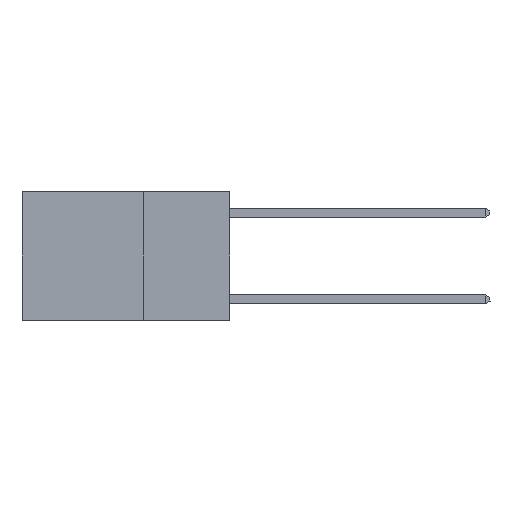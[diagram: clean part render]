
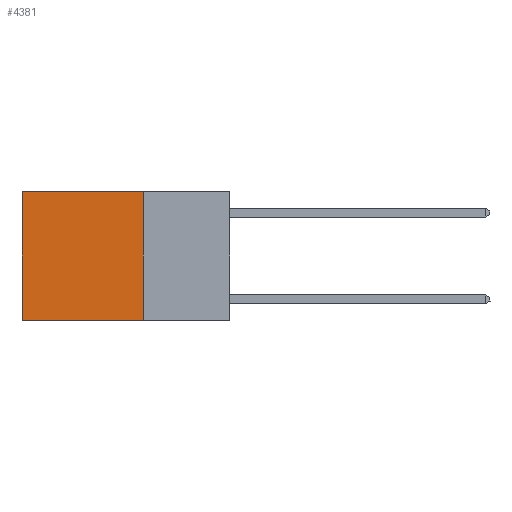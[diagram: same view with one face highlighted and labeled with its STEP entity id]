
A CAD part, left-side view. The second image highlights one B-rep face of the part: STEP entity #4381.
In plain terms, the highlighted planar face has unit normal (-1, 0, 0).
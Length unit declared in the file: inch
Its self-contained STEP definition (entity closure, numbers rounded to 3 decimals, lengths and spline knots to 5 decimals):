
#1529 = LINE ( 'NONE', #4087, #15041 ) ;
#1538 = VERTEX_POINT ( 'NONE', #12390 ) ;
#1832 = EDGE_CURVE ( 'NONE', #18325, #11572, #9475, .T. ) ;
#1994 = DIRECTION ( 'NONE',  ( 0., 0., -1. ) ) ;
#3915 = EDGE_LOOP ( 'NONE', ( #21281, #9006, #17291, #7920 ) ) ;
#4087 = CARTESIAN_POINT ( 'NONE',  ( 0.2625, 0.25, 0. ) ) ;
#4342 = CARTESIAN_POINT ( 'NONE',  ( 0.2625, 0.25, -0.37 ) ) ;
#4381 = ADVANCED_FACE ( 'NONE', ( #10712 ), #11889, .F. ) ;
#5297 = EDGE_CURVE ( 'NONE', #1538, #17849, #1529, .T. ) ;
#5968 = DIRECTION ( 'NONE',  ( 1., 0., 0. ) ) ;
#6280 = CARTESIAN_POINT ( 'NONE',  ( 0.2625, 0.25, -0.37 ) ) ;
#6551 = AXIS2_PLACEMENT_3D ( 'NONE', #14494, #5968, #1994 ) ;
#7920 = ORIENTED_EDGE ( 'NONE', *, *, #5297, .T. ) ;
#8120 = VECTOR ( 'NONE', #9567, 39.37008 ) ;
#9006 = ORIENTED_EDGE ( 'NONE', *, *, #1832, .F. ) ;
#9340 = LINE ( 'NONE', #21390, #16063 ) ;
#9475 = LINE ( 'NONE', #4342, #8120 ) ;
#9567 = DIRECTION ( 'NONE',  ( 0., 1., 0. ) ) ;
#10415 = CARTESIAN_POINT ( 'NONE',  ( 0.2625, 0.6, 0. ) ) ;
#10712 = FACE_OUTER_BOUND ( 'NONE', #3915, .T. ) ;
#10870 = VECTOR ( 'NONE', #11507, 39.37008 ) ;
#11131 = CARTESIAN_POINT ( 'NONE',  ( 0.2625, 0.6, -0.37 ) ) ;
#11487 = DIRECTION ( 'NONE',  ( 0., 0., -1. ) ) ;
#11507 = DIRECTION ( 'NONE',  ( 0., 0., -1. ) ) ;
#11572 = VERTEX_POINT ( 'NONE', #11131 ) ;
#11889 = PLANE ( 'NONE',  #6551 ) ;
#12390 = CARTESIAN_POINT ( 'NONE',  ( 0.2625, 0.25, 0. ) ) ;
#14466 = DIRECTION ( 'NONE',  ( 0., 1., 0. ) ) ;
#14494 = CARTESIAN_POINT ( 'NONE',  ( 0.2625, 0.25, 0. ) ) ;
#14552 = EDGE_CURVE ( 'NONE', #17849, #11572, #9340, .T. ) ;
#15041 = VECTOR ( 'NONE', #14466, 39.37008 ) ;
#16063 = VECTOR ( 'NONE', #11487, 39.37008 ) ;
#16964 = EDGE_CURVE ( 'NONE', #1538, #18325, #21074, .T. ) ;
#17291 = ORIENTED_EDGE ( 'NONE', *, *, #16964, .F. ) ;
#17849 = VERTEX_POINT ( 'NONE', #10415 ) ;
#18325 = VERTEX_POINT ( 'NONE', #6280 ) ;
#21074 = LINE ( 'NONE', #21842, #10870 ) ;
#21281 = ORIENTED_EDGE ( 'NONE', *, *, #14552, .T. ) ;
#21390 = CARTESIAN_POINT ( 'NONE',  ( 0.2625, 0.6, 0. ) ) ;
#21842 = CARTESIAN_POINT ( 'NONE',  ( 0.2625, 0.25, 0. ) ) ;
